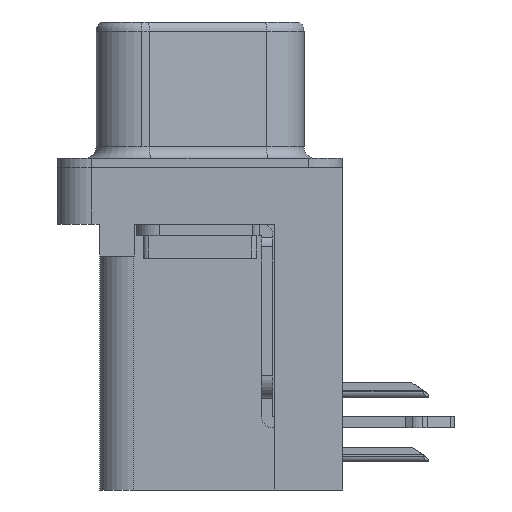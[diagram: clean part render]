
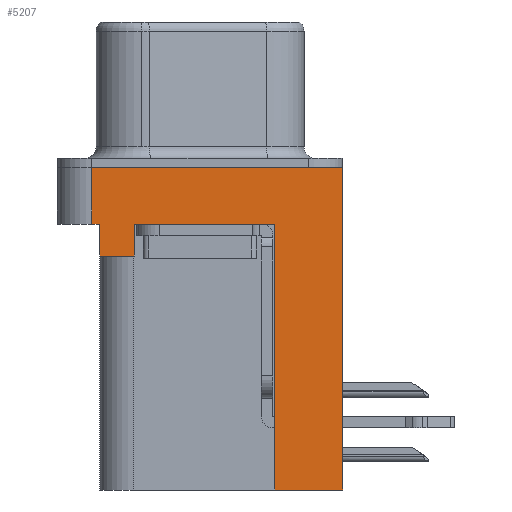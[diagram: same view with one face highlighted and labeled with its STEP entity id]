
A CAD part, left-side view. The second image highlights one B-rep face of the part: STEP entity #5207.
In plain terms, the highlighted planar face has unit normal (-1, 0, 0).
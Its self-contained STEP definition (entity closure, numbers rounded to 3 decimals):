
#557 = VECTOR ( 'NONE', #1866, 1000. ) ;
#843 = CARTESIAN_POINT ( 'NONE',  ( -3., -6.275, -2.5 ) ) ;
#859 = DIRECTION ( 'NONE',  ( 0., 0., 1. ) ) ;
#1258 = EDGE_CURVE ( 'NONE', #2137, #8988, #19878, .T. ) ;
#1866 = DIRECTION ( 'NONE',  ( 0., -1., 0. ) ) ;
#2137 = VERTEX_POINT ( 'NONE', #16696 ) ;
#3117 = ORIENTED_EDGE ( 'NONE', *, *, #13365, .F. ) ;
#3141 = CARTESIAN_POINT ( 'NONE',  ( -3., -6.275, -2.5 ) ) ;
#3881 = ORIENTED_EDGE ( 'NONE', *, *, #8953, .F. ) ;
#4022 = CARTESIAN_POINT ( 'NONE',  ( -3., 2.895, -3.9 ) ) ;
#4341 = VECTOR ( 'NONE', #20101, 1000. ) ;
#4364 = VECTOR ( 'NONE', #10376, 1000. ) ;
#4431 = VECTOR ( 'NONE', #6544, 1000. ) ;
#4950 = VERTEX_POINT ( 'NONE', #16119 ) ;
#5072 = EDGE_CURVE ( 'NONE', #5734, #15662, #15054, .T. ) ;
#5207 = ADVANCED_FACE ( 'NONE', ( #10410 ), #19337, .T. ) ;
#5734 = VERTEX_POINT ( 'NONE', #11713 ) ;
#6022 = CARTESIAN_POINT ( 'NONE',  ( -3., 4.775, -2.5 ) ) ;
#6323 = CARTESIAN_POINT ( 'NONE',  ( -3., -6.275, 0. ) ) ;
#6504 = EDGE_CURVE ( 'NONE', #8323, #10581, #7735, .T. ) ;
#6544 = DIRECTION ( 'NONE',  ( 0., 0., 1. ) ) ;
#6662 = ORIENTED_EDGE ( 'NONE', *, *, #1258, .T. ) ;
#7014 = VECTOR ( 'NONE', #17843, 1000. ) ;
#7199 = EDGE_CURVE ( 'NONE', #10581, #4950, #15681, .T. ) ;
#7273 = CARTESIAN_POINT ( 'NONE',  ( -3., -6.275, -2.5 ) ) ;
#7289 = LINE ( 'NONE', #10771, #7014 ) ;
#7735 = LINE ( 'NONE', #4022, #13707 ) ;
#8209 = ORIENTED_EDGE ( 'NONE', *, *, #13163, .F. ) ;
#8323 = VERTEX_POINT ( 'NONE', #21905 ) ;
#8881 = EDGE_CURVE ( 'NONE', #5734, #19309, #9578, .T. ) ;
#8953 = EDGE_CURVE ( 'NONE', #13358, #4950, #13407, .T. ) ;
#8988 = VERTEX_POINT ( 'NONE', #6323 ) ;
#9236 = VECTOR ( 'NONE', #11325, 1000. ) ;
#9578 = LINE ( 'NONE', #7273, #10634 ) ;
#9698 = CARTESIAN_POINT ( 'NONE',  ( -3., -3.295, -14.2 ) ) ;
#9986 = CARTESIAN_POINT ( 'NONE',  ( -3., 4.775, 0. ) ) ;
#10134 = LINE ( 'NONE', #13613, #4431 ) ;
#10376 = DIRECTION ( 'NONE',  ( 0., 1., 0. ) ) ;
#10410 = FACE_OUTER_BOUND ( 'NONE', #10945, .T. ) ;
#10529 = DIRECTION ( 'NONE',  ( -1., 0., 0. ) ) ;
#10581 = VERTEX_POINT ( 'NONE', #14774 ) ;
#10634 = VECTOR ( 'NONE', #14339, 1000. ) ;
#10771 = CARTESIAN_POINT ( 'NONE',  ( -3., 4.425, -3.9 ) ) ;
#10945 = EDGE_LOOP ( 'NONE', ( #3117, #13458, #16838, #20710, #8209, #15735, #11963, #3881, #15687, #6662 ) ) ;
#11325 = DIRECTION ( 'NONE',  ( 0., -1., 0. ) ) ;
#11436 = CARTESIAN_POINT ( 'NONE',  ( -3., -3.295, -14.2 ) ) ;
#11571 = EDGE_CURVE ( 'NONE', #2137, #13358, #12115, .T. ) ;
#11713 = CARTESIAN_POINT ( 'NONE',  ( -3., 4.775, -2.5 ) ) ;
#11963 = ORIENTED_EDGE ( 'NONE', *, *, #7199, .T. ) ;
#12115 = LINE ( 'NONE', #22796, #4364 ) ;
#12853 = VECTOR ( 'NONE', #859, 1000. ) ;
#12962 = DIRECTION ( 'NONE',  ( 0., 0., 1. ) ) ;
#13098 = DIRECTION ( 'NONE',  ( 0., 0., 1. ) ) ;
#13163 = EDGE_CURVE ( 'NONE', #8323, #15551, #7289, .T. ) ;
#13358 = VERTEX_POINT ( 'NONE', #11436 ) ;
#13365 = EDGE_CURVE ( 'NONE', #15662, #8988, #16552, .T. ) ;
#13407 = LINE ( 'NONE', #9698, #12853 ) ;
#13458 = ORIENTED_EDGE ( 'NONE', *, *, #5072, .F. ) ;
#13613 = CARTESIAN_POINT ( 'NONE',  ( -3., 4.425, -3.9 ) ) ;
#13707 = VECTOR ( 'NONE', #12962, 1000. ) ;
#13831 = EDGE_CURVE ( 'NONE', #15551, #19309, #10134, .T. ) ;
#14339 = DIRECTION ( 'NONE',  ( 0., -1., 0. ) ) ;
#14774 = CARTESIAN_POINT ( 'NONE',  ( -3., 2.895, -2.5 ) ) ;
#14812 = CARTESIAN_POINT ( 'NONE',  ( -3., -6.275, 0. ) ) ;
#14879 = CARTESIAN_POINT ( 'NONE',  ( -3., 4.425, -3.9 ) ) ;
#15054 = LINE ( 'NONE', #6022, #16272 ) ;
#15551 = VERTEX_POINT ( 'NONE', #14879 ) ;
#15662 = VERTEX_POINT ( 'NONE', #9986 ) ;
#15681 = LINE ( 'NONE', #3141, #557 ) ;
#15687 = ORIENTED_EDGE ( 'NONE', *, *, #11571, .F. ) ;
#15735 = ORIENTED_EDGE ( 'NONE', *, *, #6504, .T. ) ;
#16119 = CARTESIAN_POINT ( 'NONE',  ( -3., -3.295, -2.5 ) ) ;
#16272 = VECTOR ( 'NONE', #13098, 1000. ) ;
#16552 = LINE ( 'NONE', #14812, #9236 ) ;
#16696 = CARTESIAN_POINT ( 'NONE',  ( -3., -6.275, -14.2 ) ) ;
#16794 = CARTESIAN_POINT ( 'NONE',  ( -3., 4.425, -2.5 ) ) ;
#16838 = ORIENTED_EDGE ( 'NONE', *, *, #8881, .T. ) ;
#17604 = DIRECTION ( 'NONE',  ( 0., 0., 1. ) ) ;
#17714 = AXIS2_PLACEMENT_3D ( 'NONE', #20730, #10529, #17604 ) ;
#17843 = DIRECTION ( 'NONE',  ( 0., 1., 0. ) ) ;
#19309 = VERTEX_POINT ( 'NONE', #16794 ) ;
#19337 = PLANE ( 'NONE',  #17714 ) ;
#19878 = LINE ( 'NONE', #843, #4341 ) ;
#20101 = DIRECTION ( 'NONE',  ( 0., 0., 1. ) ) ;
#20710 = ORIENTED_EDGE ( 'NONE', *, *, #13831, .F. ) ;
#20730 = CARTESIAN_POINT ( 'NONE',  ( -3., -6.275, -2.5 ) ) ;
#21905 = CARTESIAN_POINT ( 'NONE',  ( -3., 2.895, -3.9 ) ) ;
#22796 = CARTESIAN_POINT ( 'NONE',  ( -3., -3.295, -14.2 ) ) ;
